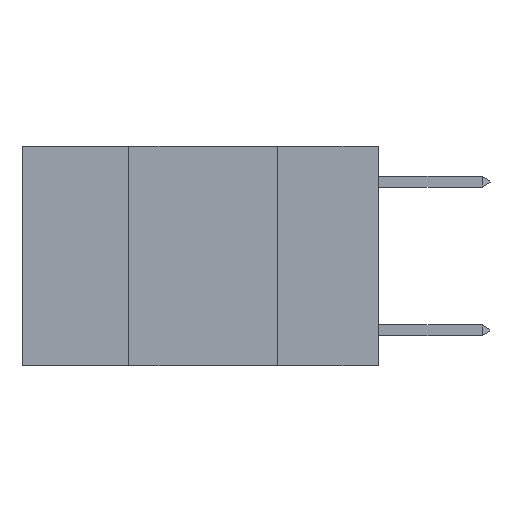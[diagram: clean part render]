
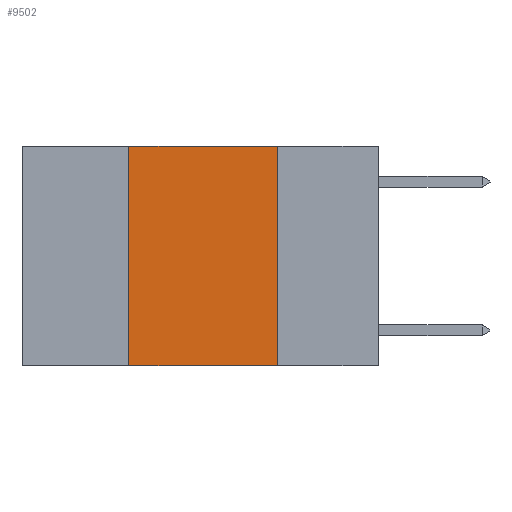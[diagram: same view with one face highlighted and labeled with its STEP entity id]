
A CAD part, left-side view. The second image highlights one B-rep face of the part: STEP entity #9502.
In plain terms, the highlighted planar face has unit normal (-1, 0, 0).
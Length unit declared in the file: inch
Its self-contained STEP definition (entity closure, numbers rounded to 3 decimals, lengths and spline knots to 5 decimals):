
#837 = CARTESIAN_POINT ( 'NONE',  ( 0., 0.17, -0.37 ) ) ;
#955 = EDGE_CURVE ( 'NONE', #4319, #1448, #14204, .T. ) ;
#1115 = EDGE_CURVE ( 'NONE', #18501, #4319, #17072, .T. ) ;
#1356 = LINE ( 'NONE', #7764, #10438 ) ;
#1448 = VERTEX_POINT ( 'NONE', #12714 ) ;
#1493 = EDGE_CURVE ( 'NONE', #18501, #19940, #1356, .T. ) ;
#1707 = DIRECTION ( 'NONE',  ( 0., -1., 0. ) ) ;
#2330 = DIRECTION ( 'NONE',  ( 0., 0., 1. ) ) ;
#3563 = LINE ( 'NONE', #13002, #12706 ) ;
#4319 = VERTEX_POINT ( 'NONE', #17057 ) ;
#4591 = EDGE_CURVE ( 'NONE', #1448, #19940, #3563, .T. ) ;
#4949 = ORIENTED_EDGE ( 'NONE', *, *, #1115, .F. ) ;
#6007 = DIRECTION ( 'NONE',  ( 0., -1., 0. ) ) ;
#7383 = ORIENTED_EDGE ( 'NONE', *, *, #4591, .F. ) ;
#7764 = CARTESIAN_POINT ( 'NONE',  ( 0., 0.6, -0.37 ) ) ;
#9498 = DIRECTION ( 'NONE',  ( 1., 0., 0. ) ) ;
#9502 = ADVANCED_FACE ( 'NONE', ( #19119 ), #11060, .F. ) ;
#9707 = CARTESIAN_POINT ( 'NONE',  ( 0., 0.6, 0. ) ) ;
#10141 = DIRECTION ( 'NONE',  ( 0., 0., -1. ) ) ;
#10438 = VECTOR ( 'NONE', #6007, 39.37008 ) ;
#10712 = AXIS2_PLACEMENT_3D ( 'NONE', #9707, #9498, #15910 ) ;
#11060 = PLANE ( 'NONE',  #10712 ) ;
#11862 = EDGE_LOOP ( 'NONE', ( #7383, #12977, #4949, #14356 ) ) ;
#12706 = VECTOR ( 'NONE', #10141, 39.37008 ) ;
#12714 = CARTESIAN_POINT ( 'NONE',  ( 0., 0.17, 0. ) ) ;
#12956 = CARTESIAN_POINT ( 'NONE',  ( 0., 0.6, 0. ) ) ;
#12977 = ORIENTED_EDGE ( 'NONE', *, *, #955, .F. ) ;
#13002 = CARTESIAN_POINT ( 'NONE',  ( 0., 0.17, 0. ) ) ;
#14204 = LINE ( 'NONE', #12956, #14808 ) ;
#14356 = ORIENTED_EDGE ( 'NONE', *, *, #1493, .T. ) ;
#14808 = VECTOR ( 'NONE', #1707, 39.37008 ) ;
#15910 = DIRECTION ( 'NONE',  ( 0., 0., -1. ) ) ;
#17057 = CARTESIAN_POINT ( 'NONE',  ( 0., 0.42, 0. ) ) ;
#17072 = LINE ( 'NONE', #20053, #18224 ) ;
#17261 = CARTESIAN_POINT ( 'NONE',  ( 0., 0.42, -0.37 ) ) ;
#18224 = VECTOR ( 'NONE', #2330, 39.37008 ) ;
#18501 = VERTEX_POINT ( 'NONE', #17261 ) ;
#19119 = FACE_OUTER_BOUND ( 'NONE', #11862, .T. ) ;
#19940 = VERTEX_POINT ( 'NONE', #837 ) ;
#20053 = CARTESIAN_POINT ( 'NONE',  ( 0., 0.42, 0. ) ) ;
